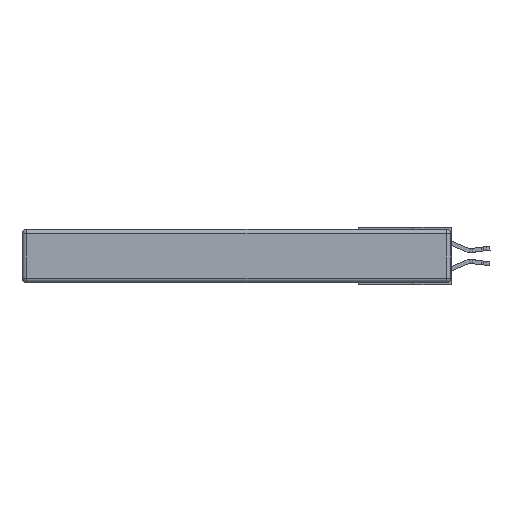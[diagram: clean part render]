
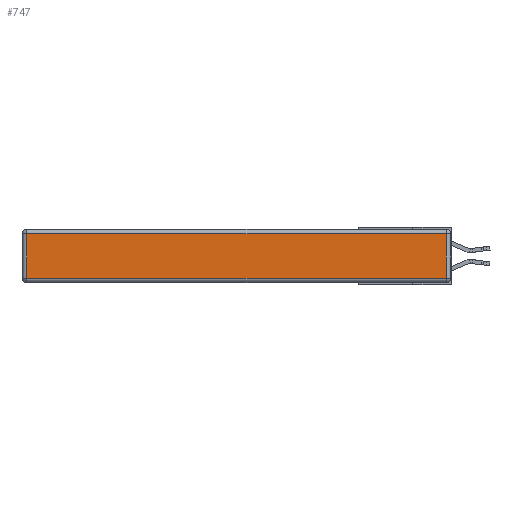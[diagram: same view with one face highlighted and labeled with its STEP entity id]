
A CAD part, left-side view. The second image highlights one B-rep face of the part: STEP entity #747.
In plain terms, the highlighted planar face has unit normal (-1, 0, 0).
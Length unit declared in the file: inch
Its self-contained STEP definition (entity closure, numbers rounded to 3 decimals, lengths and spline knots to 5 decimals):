
#747 = ADVANCED_FACE ( 'NONE', ( #20838 ), #21340, .T. ) ;
#1111 = ORIENTED_EDGE ( 'NONE', *, *, #3854, .T. ) ;
#2653 = CARTESIAN_POINT ( 'NONE',  ( 0., 2.75, -0.03 ) ) ;
#2791 = VERTEX_POINT ( 'NONE', #33554 ) ;
#2959 = VECTOR ( 'NONE', #33141, 39.37008 ) ;
#3854 = EDGE_CURVE ( 'NONE', #24248, #2791, #11468, .T. ) ;
#5255 = VECTOR ( 'NONE', #28660, 39.37008 ) ;
#5714 = CARTESIAN_POINT ( 'NONE',  ( 0., 2.72, -0.313 ) ) ;
#7893 = CARTESIAN_POINT ( 'NONE',  ( 0., 0.03, -0.03 ) ) ;
#11050 = VECTOR ( 'NONE', #18711, 39.37008 ) ;
#11324 = AXIS2_PLACEMENT_3D ( 'NONE', #26558, #16007, #18903 ) ;
#11468 = LINE ( 'NONE', #2653, #5255 ) ;
#13230 = CARTESIAN_POINT ( 'NONE',  ( 0., 0.03, -0.343 ) ) ;
#13733 = EDGE_LOOP ( 'NONE', ( #21001, #18005, #1111, #26284 ) ) ;
#13742 = LINE ( 'NONE', #30596, #2959 ) ;
#14776 = DIRECTION ( 'NONE',  ( 0., -1., 0. ) ) ;
#16007 = DIRECTION ( 'NONE',  ( -1., 0., 0. ) ) ;
#16465 = LINE ( 'NONE', #13230, #11050 ) ;
#17048 = VECTOR ( 'NONE', #14776, 39.37008 ) ;
#18005 = ORIENTED_EDGE ( 'NONE', *, *, #19629, .T. ) ;
#18711 = DIRECTION ( 'NONE',  ( 0., 0., 1. ) ) ;
#18903 = DIRECTION ( 'NONE',  ( 0., 0., 1. ) ) ;
#19629 = EDGE_CURVE ( 'NONE', #22082, #24248, #16465, .T. ) ;
#20838 = FACE_OUTER_BOUND ( 'NONE', #13733, .T. ) ;
#21001 = ORIENTED_EDGE ( 'NONE', *, *, #23915, .T. ) ;
#21340 = PLANE ( 'NONE',  #11324 ) ;
#22082 = VERTEX_POINT ( 'NONE', #28911 ) ;
#23150 = EDGE_CURVE ( 'NONE', #2791, #29853, #13742, .T. ) ;
#23915 = EDGE_CURVE ( 'NONE', #29853, #22082, #24101, .T. ) ;
#24101 = LINE ( 'NONE', #30438, #17048 ) ;
#24248 = VERTEX_POINT ( 'NONE', #7893 ) ;
#26284 = ORIENTED_EDGE ( 'NONE', *, *, #23150, .T. ) ;
#26558 = CARTESIAN_POINT ( 'NONE',  ( 0., 0., -0.343 ) ) ;
#28660 = DIRECTION ( 'NONE',  ( 0., 1., 0. ) ) ;
#28911 = CARTESIAN_POINT ( 'NONE',  ( 0., 0.03, -0.313 ) ) ;
#29853 = VERTEX_POINT ( 'NONE', #5714 ) ;
#30438 = CARTESIAN_POINT ( 'NONE',  ( 0., 0., -0.313 ) ) ;
#30596 = CARTESIAN_POINT ( 'NONE',  ( 0., 2.72, -0.343 ) ) ;
#33141 = DIRECTION ( 'NONE',  ( 0., 0., -1. ) ) ;
#33554 = CARTESIAN_POINT ( 'NONE',  ( 0., 2.72, -0.03 ) ) ;
